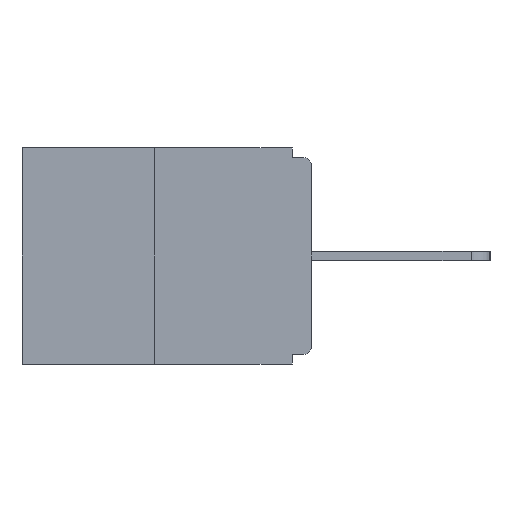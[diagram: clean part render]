
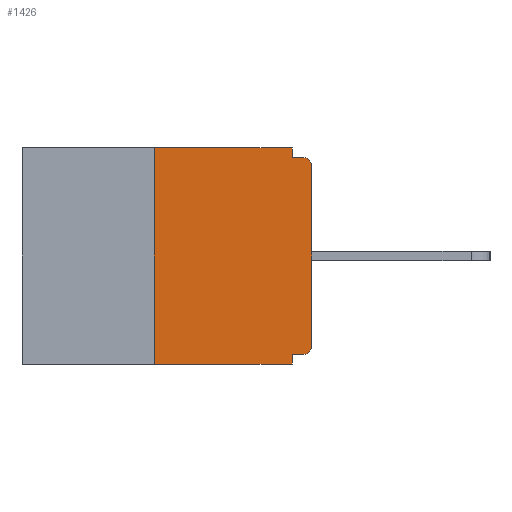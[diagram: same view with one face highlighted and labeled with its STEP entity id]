
A CAD part, left-side view. The second image highlights one B-rep face of the part: STEP entity #1426.
In plain terms, the highlighted planar face has unit normal (-1, 0, 0).
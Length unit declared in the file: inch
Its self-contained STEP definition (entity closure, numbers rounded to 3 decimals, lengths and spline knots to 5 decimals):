
#57 = ORIENTED_EDGE ( 'NONE', *, *, #674, .F. ) ;
#636 = DIRECTION ( 'NONE',  ( 0., -1., 0. ) ) ;
#639 = VECTOR ( 'NONE', #7592, 39.37008 ) ;
#674 = EDGE_CURVE ( 'NONE', #10157, #18696, #6343, .T. ) ;
#792 = DIRECTION ( 'NONE',  ( 0., 0., -1. ) ) ;
#965 = LINE ( 'NONE', #16985, #17460 ) ;
#1426 = ADVANCED_FACE ( 'NONE', ( #9835 ), #11136, .F. ) ;
#1696 = CIRCLE ( 'NONE', #8111, 0.015 ) ;
#2106 = VERTEX_POINT ( 'NONE', #7001 ) ;
#2138 = CARTESIAN_POINT ( 'NONE',  ( 0., 0.46, -0.343 ) ) ;
#2208 = DIRECTION ( 'NONE',  ( -1., 0., 0. ) ) ;
#2394 = CARTESIAN_POINT ( 'NONE',  ( 0., 0.015, -0.313 ) ) ;
#2542 = ORIENTED_EDGE ( 'NONE', *, *, #5445, .F. ) ;
#2711 = VECTOR ( 'NONE', #636, 39.37008 ) ;
#2895 = DIRECTION ( 'NONE',  ( 0., 0., -1. ) ) ;
#3027 = ORIENTED_EDGE ( 'NONE', *, *, #17516, .F. ) ;
#3115 = VECTOR ( 'NONE', #7196, 39.37008 ) ;
#3724 = DIRECTION ( 'NONE',  ( 0., 0., -1. ) ) ;
#4143 = EDGE_CURVE ( 'NONE', #14753, #8166, #16685, .T. ) ;
#4709 = VERTEX_POINT ( 'NONE', #11624 ) ;
#4910 = EDGE_LOOP ( 'NONE', ( #6490, #57, #8509, #9022, #13121, #9535, #17544, #6244, #2542, #3027 ) ) ;
#5139 = EDGE_CURVE ( 'NONE', #18696, #6705, #6037, .T. ) ;
#5196 = CARTESIAN_POINT ( 'NONE',  ( 0., 0., -0.328 ) ) ;
#5445 = EDGE_CURVE ( 'NONE', #4709, #16511, #9554, .T. ) ;
#5942 = CARTESIAN_POINT ( 'NONE',  ( 0., 0.031, 0. ) ) ;
#6037 = LINE ( 'NONE', #18439, #14360 ) ;
#6212 = CARTESIAN_POINT ( 'NONE',  ( 0., 0.25, -0.343 ) ) ;
#6244 = ORIENTED_EDGE ( 'NONE', *, *, #18529, .T. ) ;
#6343 = LINE ( 'NONE', #6942, #3115 ) ;
#6426 = CARTESIAN_POINT ( 'NONE',  ( 0., 0., -0.015 ) ) ;
#6438 = CARTESIAN_POINT ( 'NONE',  ( 0., 0., -0.313 ) ) ;
#6490 = ORIENTED_EDGE ( 'NONE', *, *, #5139, .F. ) ;
#6705 = VERTEX_POINT ( 'NONE', #5942 ) ;
#6942 = CARTESIAN_POINT ( 'NONE',  ( 0., 0.25, 0. ) ) ;
#7001 = CARTESIAN_POINT ( 'NONE',  ( 0., 0.031, -0.343 ) ) ;
#7196 = DIRECTION ( 'NONE',  ( 0., 0., 1. ) ) ;
#7367 = CARTESIAN_POINT ( 'NONE',  ( 0., 0.031, 0. ) ) ;
#7592 = DIRECTION ( 'NONE',  ( 0., 1., 0. ) ) ;
#7740 = DIRECTION ( 'NONE',  ( 0., -1., 0. ) ) ;
#8111 = AXIS2_PLACEMENT_3D ( 'NONE', #2394, #2208, #2895 ) ;
#8166 = VERTEX_POINT ( 'NONE', #9800 ) ;
#8509 = ORIENTED_EDGE ( 'NONE', *, *, #19067, .T. ) ;
#8560 = EDGE_CURVE ( 'NONE', #14753, #14036, #1696, .T. ) ;
#9022 = ORIENTED_EDGE ( 'NONE', *, *, #9851, .F. ) ;
#9047 = VECTOR ( 'NONE', #7740, 39.37008 ) ;
#9535 = ORIENTED_EDGE ( 'NONE', *, *, #8560, .T. ) ;
#9554 = LINE ( 'NONE', #6426, #9047 ) ;
#9800 = CARTESIAN_POINT ( 'NONE',  ( 0., 0.031, -0.328 ) ) ;
#9835 = FACE_OUTER_BOUND ( 'NONE', #4910, .T. ) ;
#9851 = EDGE_CURVE ( 'NONE', #8166, #2106, #11091, .T. ) ;
#10157 = VERTEX_POINT ( 'NONE', #6212 ) ;
#10328 = DIRECTION ( 'NONE',  ( -1., 0., 0. ) ) ;
#10338 = CARTESIAN_POINT ( 'NONE',  ( 0., 0.015, -0.328 ) ) ;
#10718 = LINE ( 'NONE', #7367, #13821 ) ;
#10795 = DIRECTION ( 'NONE',  ( 0., 0., -1. ) ) ;
#10957 = DIRECTION ( 'NONE',  ( 0., 0., 1. ) ) ;
#11091 = LINE ( 'NONE', #14742, #19083 ) ;
#11136 = PLANE ( 'NONE',  #16981 ) ;
#11150 = LINE ( 'NONE', #2138, #2711 ) ;
#11624 = CARTESIAN_POINT ( 'NONE',  ( 0., 0.031, -0.015 ) ) ;
#12039 = DIRECTION ( 'NONE',  ( 1., 0., 0. ) ) ;
#12171 = VERTEX_POINT ( 'NONE', #16247 ) ;
#12206 = CARTESIAN_POINT ( 'NONE',  ( 0., 0.46, 0. ) ) ;
#12335 = CARTESIAN_POINT ( 'NONE',  ( 0., 0.015, -0.015 ) ) ;
#13121 = ORIENTED_EDGE ( 'NONE', *, *, #4143, .F. ) ;
#13821 = VECTOR ( 'NONE', #16550, 39.37008 ) ;
#14036 = VERTEX_POINT ( 'NONE', #6438 ) ;
#14360 = VECTOR ( 'NONE', #18397, 39.37008 ) ;
#14742 = CARTESIAN_POINT ( 'NONE',  ( 0., 0.031, -0.343 ) ) ;
#14753 = VERTEX_POINT ( 'NONE', #10338 ) ;
#14958 = AXIS2_PLACEMENT_3D ( 'NONE', #19342, #10328, #792 ) ;
#16247 = CARTESIAN_POINT ( 'NONE',  ( 0., 0., -0.03 ) ) ;
#16296 = CIRCLE ( 'NONE', #14958, 0.015 ) ;
#16511 = VERTEX_POINT ( 'NONE', #12335 ) ;
#16550 = DIRECTION ( 'NONE',  ( 0., 0., -1. ) ) ;
#16685 = LINE ( 'NONE', #5196, #639 ) ;
#16981 = AXIS2_PLACEMENT_3D ( 'NONE', #12206, #12039, #10795 ) ;
#16985 = CARTESIAN_POINT ( 'NONE',  ( 0., 0., 0. ) ) ;
#17460 = VECTOR ( 'NONE', #10957, 39.37008 ) ;
#17516 = EDGE_CURVE ( 'NONE', #6705, #4709, #10718, .T. ) ;
#17544 = ORIENTED_EDGE ( 'NONE', *, *, #19388, .T. ) ;
#18397 = DIRECTION ( 'NONE',  ( 0., -1., 0. ) ) ;
#18439 = CARTESIAN_POINT ( 'NONE',  ( 0., 0.46, 0. ) ) ;
#18529 = EDGE_CURVE ( 'NONE', #12171, #16511, #16296, .T. ) ;
#18696 = VERTEX_POINT ( 'NONE', #19726 ) ;
#19067 = EDGE_CURVE ( 'NONE', #10157, #2106, #11150, .T. ) ;
#19083 = VECTOR ( 'NONE', #3724, 39.37008 ) ;
#19342 = CARTESIAN_POINT ( 'NONE',  ( 0., 0.015, -0.03 ) ) ;
#19388 = EDGE_CURVE ( 'NONE', #14036, #12171, #965, .T. ) ;
#19726 = CARTESIAN_POINT ( 'NONE',  ( 0., 0.25, 0. ) ) ;
